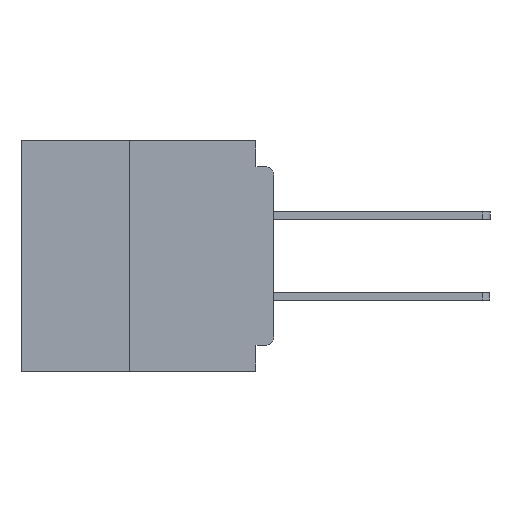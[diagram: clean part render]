
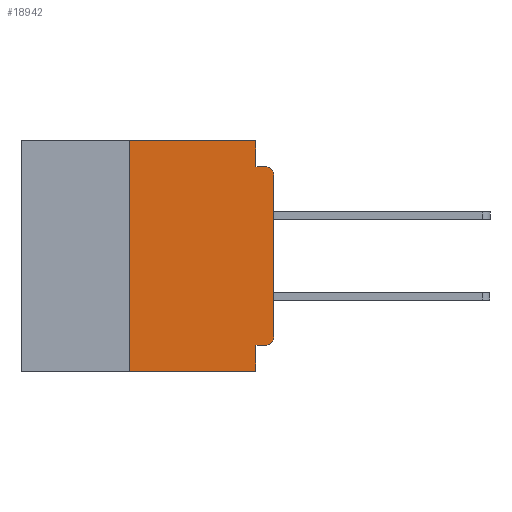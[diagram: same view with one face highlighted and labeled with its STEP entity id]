
A CAD part, left-side view. The second image highlights one B-rep face of the part: STEP entity #18942.
In plain terms, the highlighted planar face has unit normal (-1, 0, 0).
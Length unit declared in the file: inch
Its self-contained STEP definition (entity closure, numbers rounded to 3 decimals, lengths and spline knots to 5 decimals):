
#1238 = DIRECTION ( 'NONE',  ( 0., 0., -1. ) ) ;
#1338 = VERTEX_POINT ( 'NONE', #6978 ) ;
#1895 = VECTOR ( 'NONE', #27401, 39.37008 ) ;
#1963 = EDGE_CURVE ( 'NONE', #38453, #7329, #41503, .T. ) ;
#2214 = ORIENTED_EDGE ( 'NONE', *, *, #42297, .F. ) ;
#3776 = EDGE_CURVE ( 'NONE', #7556, #14695, #4566, .T. ) ;
#4387 = CARTESIAN_POINT ( 'NONE',  ( 0., 0.031, -0.045 ) ) ;
#4525 = AXIS2_PLACEMENT_3D ( 'NONE', #13129, #36413, #16473 ) ;
#4566 = LINE ( 'NONE', #42622, #12545 ) ;
#5036 = ORIENTED_EDGE ( 'NONE', *, *, #1963, .F. ) ;
#6298 = DIRECTION ( 'NONE',  ( 0., -1., 0. ) ) ;
#6978 = CARTESIAN_POINT ( 'NONE',  ( 0., 0.015, -0.355 ) ) ;
#7279 = VECTOR ( 'NONE', #18116, 39.37008 ) ;
#7329 = VERTEX_POINT ( 'NONE', #7373 ) ;
#7373 = CARTESIAN_POINT ( 'NONE',  ( 0., 0.031, -0.4 ) ) ;
#7393 = DIRECTION ( 'NONE',  ( 0., 0., 1. ) ) ;
#7556 = VERTEX_POINT ( 'NONE', #9015 ) ;
#8149 = LINE ( 'NONE', #41256, #33719 ) ;
#9015 = CARTESIAN_POINT ( 'NONE',  ( 0., 0.25, 0. ) ) ;
#9420 = ORIENTED_EDGE ( 'NONE', *, *, #19503, .F. ) ;
#9625 = CIRCLE ( 'NONE', #4525, 0.015 ) ;
#10593 = VECTOR ( 'NONE', #7393, 39.37008 ) ;
#11010 = EDGE_CURVE ( 'NONE', #19224, #21030, #19423, .T. ) ;
#11560 = ORIENTED_EDGE ( 'NONE', *, *, #3776, .F. ) ;
#11569 = VECTOR ( 'NONE', #16548, 39.37008 ) ;
#11874 = PLANE ( 'NONE',  #32073 ) ;
#12545 = VECTOR ( 'NONE', #42736, 39.37008 ) ;
#13037 = LINE ( 'NONE', #37414, #1895 ) ;
#13056 = ORIENTED_EDGE ( 'NONE', *, *, #21751, .F. ) ;
#13069 = CARTESIAN_POINT ( 'NONE',  ( 0., 0., -0.355 ) ) ;
#13129 = CARTESIAN_POINT ( 'NONE',  ( 0., 0.015, -0.06 ) ) ;
#13979 = VECTOR ( 'NONE', #40465, 39.37008 ) ;
#13998 = CARTESIAN_POINT ( 'NONE',  ( 0., 0., 0. ) ) ;
#14695 = VERTEX_POINT ( 'NONE', #23432 ) ;
#15318 = CARTESIAN_POINT ( 'NONE',  ( 0., 0.015, -0.34 ) ) ;
#16196 = LINE ( 'NONE', #28039, #7279 ) ;
#16333 = ORIENTED_EDGE ( 'NONE', *, *, #18967, .T. ) ;
#16473 = DIRECTION ( 'NONE',  ( 0., 0., -1. ) ) ;
#16548 = DIRECTION ( 'NONE',  ( 0., 1., 0. ) ) ;
#18116 = DIRECTION ( 'NONE',  ( 0., 0., 1. ) ) ;
#18522 = DIRECTION ( 'NONE',  ( 1., 0., 0. ) ) ;
#18659 = DIRECTION ( 'NONE',  ( 0., 0., -1. ) ) ;
#18942 = ADVANCED_FACE ( 'NONE', ( #20650 ), #11874, .F. ) ;
#18967 = EDGE_CURVE ( 'NONE', #1338, #19224, #29541, .T. ) ;
#19051 = VECTOR ( 'NONE', #6298, 39.37008 ) ;
#19224 = VERTEX_POINT ( 'NONE', #42993 ) ;
#19423 = LINE ( 'NONE', #13998, #10593 ) ;
#19503 = EDGE_CURVE ( 'NONE', #14695, #38943, #8149, .T. ) ;
#20376 = LINE ( 'NONE', #13069, #11569 ) ;
#20439 = CARTESIAN_POINT ( 'NONE',  ( 0., 0.015, -0.045 ) ) ;
#20650 = FACE_OUTER_BOUND ( 'NONE', #25757, .T. ) ;
#21030 = VERTEX_POINT ( 'NONE', #40219 ) ;
#21662 = ORIENTED_EDGE ( 'NONE', *, *, #32205, .T. ) ;
#21751 = EDGE_CURVE ( 'NONE', #43082, #7556, #16196, .T. ) ;
#23131 = CARTESIAN_POINT ( 'NONE',  ( 0., 0., -0.045 ) ) ;
#23432 = CARTESIAN_POINT ( 'NONE',  ( 0., 0.031, 0. ) ) ;
#25420 = EDGE_CURVE ( 'NONE', #38943, #36171, #28970, .T. ) ;
#25757 = EDGE_LOOP ( 'NONE', ( #31533, #32117, #36461, #9420, #11560, #13056, #21662, #5036, #2214, #16333 ) ) ;
#27115 = CARTESIAN_POINT ( 'NONE',  ( 0., 0.25, -0.4 ) ) ;
#27401 = DIRECTION ( 'NONE',  ( 0., -1., 0. ) ) ;
#28039 = CARTESIAN_POINT ( 'NONE',  ( 0., 0.25, -0.4 ) ) ;
#28970 = LINE ( 'NONE', #23131, #19051 ) ;
#29541 = CIRCLE ( 'NONE', #34280, 0.015 ) ;
#31533 = ORIENTED_EDGE ( 'NONE', *, *, #11010, .T. ) ;
#32073 = AXIS2_PLACEMENT_3D ( 'NONE', #38448, #18522, #41730 ) ;
#32117 = ORIENTED_EDGE ( 'NONE', *, *, #40549, .T. ) ;
#32205 = EDGE_CURVE ( 'NONE', #43082, #7329, #13037, .T. ) ;
#33719 = VECTOR ( 'NONE', #1238, 39.37008 ) ;
#34280 = AXIS2_PLACEMENT_3D ( 'NONE', #15318, #38590, #18659 ) ;
#36171 = VERTEX_POINT ( 'NONE', #20439 ) ;
#36413 = DIRECTION ( 'NONE',  ( -1., 0., 0. ) ) ;
#36461 = ORIENTED_EDGE ( 'NONE', *, *, #25420, .F. ) ;
#37414 = CARTESIAN_POINT ( 'NONE',  ( 0., 0.437, -0.4 ) ) ;
#37879 = CARTESIAN_POINT ( 'NONE',  ( 0., 0.031, -0.355 ) ) ;
#38448 = CARTESIAN_POINT ( 'NONE',  ( 0., 0.437, 0. ) ) ;
#38453 = VERTEX_POINT ( 'NONE', #37879 ) ;
#38590 = DIRECTION ( 'NONE',  ( -1., 0., 0. ) ) ;
#38943 = VERTEX_POINT ( 'NONE', #4387 ) ;
#40219 = CARTESIAN_POINT ( 'NONE',  ( 0., 0., -0.06 ) ) ;
#40465 = DIRECTION ( 'NONE',  ( 0., 0., -1. ) ) ;
#40549 = EDGE_CURVE ( 'NONE', #21030, #36171, #9625, .T. ) ;
#41140 = CARTESIAN_POINT ( 'NONE',  ( 0., 0.031, -0.4 ) ) ;
#41256 = CARTESIAN_POINT ( 'NONE',  ( 0., 0.031, 0. ) ) ;
#41503 = LINE ( 'NONE', #41140, #13979 ) ;
#41730 = DIRECTION ( 'NONE',  ( 0., 0., -1. ) ) ;
#42297 = EDGE_CURVE ( 'NONE', #1338, #38453, #20376, .T. ) ;
#42622 = CARTESIAN_POINT ( 'NONE',  ( 0., 0.437, 0. ) ) ;
#42736 = DIRECTION ( 'NONE',  ( 0., -1., 0. ) ) ;
#42993 = CARTESIAN_POINT ( 'NONE',  ( 0., 0., -0.34 ) ) ;
#43082 = VERTEX_POINT ( 'NONE', #27115 ) ;
